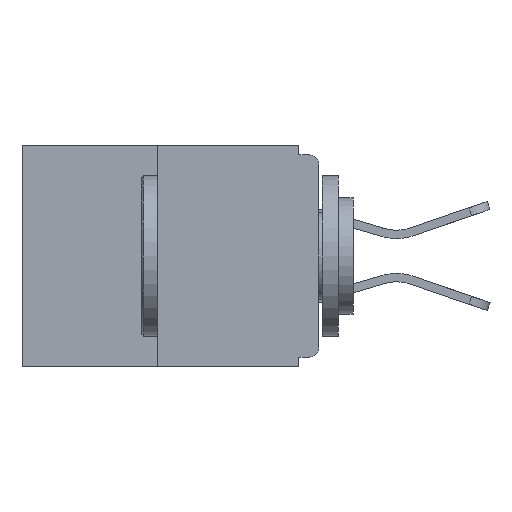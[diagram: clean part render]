
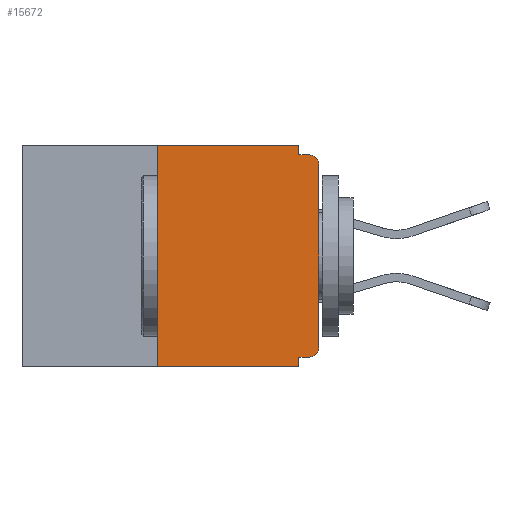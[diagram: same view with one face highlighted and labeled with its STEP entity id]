
A CAD part, left-side view. The second image highlights one B-rep face of the part: STEP entity #15672.
In plain terms, the highlighted planar face has unit normal (-1, 0, 0).
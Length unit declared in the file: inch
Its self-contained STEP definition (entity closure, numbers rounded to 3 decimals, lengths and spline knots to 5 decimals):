
#131 = CARTESIAN_POINT ( 'NONE',  ( 0., 0., -0.328 ) ) ;
#132 = CARTESIAN_POINT ( 'NONE',  ( 0., 0.015, -0.015 ) ) ;
#226 = DIRECTION ( 'NONE',  ( 0., 0., -1. ) ) ;
#667 = EDGE_LOOP ( 'NONE', ( #824, #9778, #3194, #13729, #11403, #14092, #14881, #2173, #7827, #11559 ) ) ;
#824 = ORIENTED_EDGE ( 'NONE', *, *, #2134, .F. ) ;
#1157 = CARTESIAN_POINT ( 'NONE',  ( 0., 0.031, -0.343 ) ) ;
#1419 = CARTESIAN_POINT ( 'NONE',  ( 0., 0.031, 0. ) ) ;
#1838 = CARTESIAN_POINT ( 'NONE',  ( 0., 0., -0.313 ) ) ;
#1922 = DIRECTION ( 'NONE',  ( 1., 0., 0. ) ) ;
#2047 = CARTESIAN_POINT ( 'NONE',  ( 0., 0., -0.03 ) ) ;
#2134 = EDGE_CURVE ( 'NONE', #2707, #4884, #6672, .T. ) ;
#2173 = ORIENTED_EDGE ( 'NONE', *, *, #12527, .T. ) ;
#2707 = VERTEX_POINT ( 'NONE', #11924 ) ;
#2727 = CARTESIAN_POINT ( 'NONE',  ( 0., 0.25, -0.343 ) ) ;
#2984 = CARTESIAN_POINT ( 'NONE',  ( 0., 0.015, -0.328 ) ) ;
#3067 = CARTESIAN_POINT ( 'NONE',  ( 0., 0.031, 0. ) ) ;
#3194 = ORIENTED_EDGE ( 'NONE', *, *, #16195, .T. ) ;
#3220 = VERTEX_POINT ( 'NONE', #2727 ) ;
#3250 = DIRECTION ( 'NONE',  ( -1., 0., 0. ) ) ;
#3267 = LINE ( 'NONE', #3067, #17670 ) ;
#3269 = AXIS2_PLACEMENT_3D ( 'NONE', #9029, #3250, #17558 ) ;
#3573 = CIRCLE ( 'NONE', #3269, 0.015 ) ;
#3640 = EDGE_CURVE ( 'NONE', #7118, #6739, #7491, .T. ) ;
#4038 = VERTEX_POINT ( 'NONE', #13087 ) ;
#4085 = DIRECTION ( 'NONE',  ( 0., 0., -1. ) ) ;
#4548 = EDGE_CURVE ( 'NONE', #12351, #4038, #11001, .T. ) ;
#4884 = VERTEX_POINT ( 'NONE', #1419 ) ;
#5094 = CARTESIAN_POINT ( 'NONE',  ( 0., 0.015, -0.03 ) ) ;
#6089 = VECTOR ( 'NONE', #7611, 39.37008 ) ;
#6418 = VERTEX_POINT ( 'NONE', #9271 ) ;
#6460 = DIRECTION ( 'NONE',  ( -1., 0., 0. ) ) ;
#6672 = LINE ( 'NONE', #12480, #9754 ) ;
#6739 = VERTEX_POINT ( 'NONE', #132 ) ;
#6915 = DIRECTION ( 'NONE',  ( 0., -1., 0. ) ) ;
#7085 = VECTOR ( 'NONE', #15633, 39.37008 ) ;
#7118 = VERTEX_POINT ( 'NONE', #13475 ) ;
#7367 = VERTEX_POINT ( 'NONE', #1838 ) ;
#7491 = LINE ( 'NONE', #13911, #11039 ) ;
#7611 = DIRECTION ( 'NONE',  ( 0., -1., 0. ) ) ;
#7763 = DIRECTION ( 'NONE',  ( 0., 0., -1. ) ) ;
#7827 = ORIENTED_EDGE ( 'NONE', *, *, #3640, .F. ) ;
#8629 = AXIS2_PLACEMENT_3D ( 'NONE', #17443, #1922, #11977 ) ;
#8792 = VECTOR ( 'NONE', #11478, 39.37008 ) ;
#9029 = CARTESIAN_POINT ( 'NONE',  ( 0., 0.015, -0.313 ) ) ;
#9271 = CARTESIAN_POINT ( 'NONE',  ( 0., 0.031, -0.343 ) ) ;
#9283 = CARTESIAN_POINT ( 'NONE',  ( 0., 0.25, 0. ) ) ;
#9663 = LINE ( 'NONE', #1157, #12163 ) ;
#9746 = EDGE_CURVE ( 'NONE', #12351, #7367, #3573, .T. ) ;
#9754 = VECTOR ( 'NONE', #15284, 39.37008 ) ;
#9778 = ORIENTED_EDGE ( 'NONE', *, *, #9952, .F. ) ;
#9856 = LINE ( 'NONE', #16108, #6089 ) ;
#9866 = VERTEX_POINT ( 'NONE', #2047 ) ;
#9952 = EDGE_CURVE ( 'NONE', #3220, #2707, #16199, .T. ) ;
#10090 = EDGE_CURVE ( 'NONE', #7367, #9866, #14641, .T. ) ;
#10623 = PLANE ( 'NONE',  #8629 ) ;
#11001 = LINE ( 'NONE', #131, #8792 ) ;
#11039 = VECTOR ( 'NONE', #6915, 39.37008 ) ;
#11403 = ORIENTED_EDGE ( 'NONE', *, *, #4548, .F. ) ;
#11478 = DIRECTION ( 'NONE',  ( 0., 1., 0. ) ) ;
#11559 = ORIENTED_EDGE ( 'NONE', *, *, #14032, .F. ) ;
#11678 = FACE_OUTER_BOUND ( 'NONE', #667, .T. ) ;
#11924 = CARTESIAN_POINT ( 'NONE',  ( 0., 0.25, 0. ) ) ;
#11977 = DIRECTION ( 'NONE',  ( 0., 0., -1. ) ) ;
#12163 = VECTOR ( 'NONE', #4085, 39.37008 ) ;
#12351 = VERTEX_POINT ( 'NONE', #2984 ) ;
#12461 = VECTOR ( 'NONE', #13594, 39.37008 ) ;
#12480 = CARTESIAN_POINT ( 'NONE',  ( 0., 0.46, 0. ) ) ;
#12527 = EDGE_CURVE ( 'NONE', #9866, #6739, #13276, .T. ) ;
#12820 = CARTESIAN_POINT ( 'NONE',  ( 0., 0., 0. ) ) ;
#13087 = CARTESIAN_POINT ( 'NONE',  ( 0., 0.031, -0.328 ) ) ;
#13276 = CIRCLE ( 'NONE', #15290, 0.015 ) ;
#13475 = CARTESIAN_POINT ( 'NONE',  ( 0., 0.031, -0.015 ) ) ;
#13594 = DIRECTION ( 'NONE',  ( 0., 0., 1. ) ) ;
#13729 = ORIENTED_EDGE ( 'NONE', *, *, #15360, .F. ) ;
#13911 = CARTESIAN_POINT ( 'NONE',  ( 0., 0., -0.015 ) ) ;
#14032 = EDGE_CURVE ( 'NONE', #4884, #7118, #3267, .T. ) ;
#14092 = ORIENTED_EDGE ( 'NONE', *, *, #9746, .T. ) ;
#14641 = LINE ( 'NONE', #12820, #7085 ) ;
#14881 = ORIENTED_EDGE ( 'NONE', *, *, #10090, .T. ) ;
#15284 = DIRECTION ( 'NONE',  ( 0., -1., 0. ) ) ;
#15290 = AXIS2_PLACEMENT_3D ( 'NONE', #5094, #6460, #7763 ) ;
#15360 = EDGE_CURVE ( 'NONE', #4038, #6418, #9663, .T. ) ;
#15633 = DIRECTION ( 'NONE',  ( 0., 0., 1. ) ) ;
#15672 = ADVANCED_FACE ( 'NONE', ( #11678 ), #10623, .F. ) ;
#16108 = CARTESIAN_POINT ( 'NONE',  ( 0., 0.46, -0.343 ) ) ;
#16195 = EDGE_CURVE ( 'NONE', #3220, #6418, #9856, .T. ) ;
#16199 = LINE ( 'NONE', #9283, #12461 ) ;
#17443 = CARTESIAN_POINT ( 'NONE',  ( 0., 0.46, 0. ) ) ;
#17558 = DIRECTION ( 'NONE',  ( 0., 0., -1. ) ) ;
#17670 = VECTOR ( 'NONE', #226, 39.37008 ) ;
